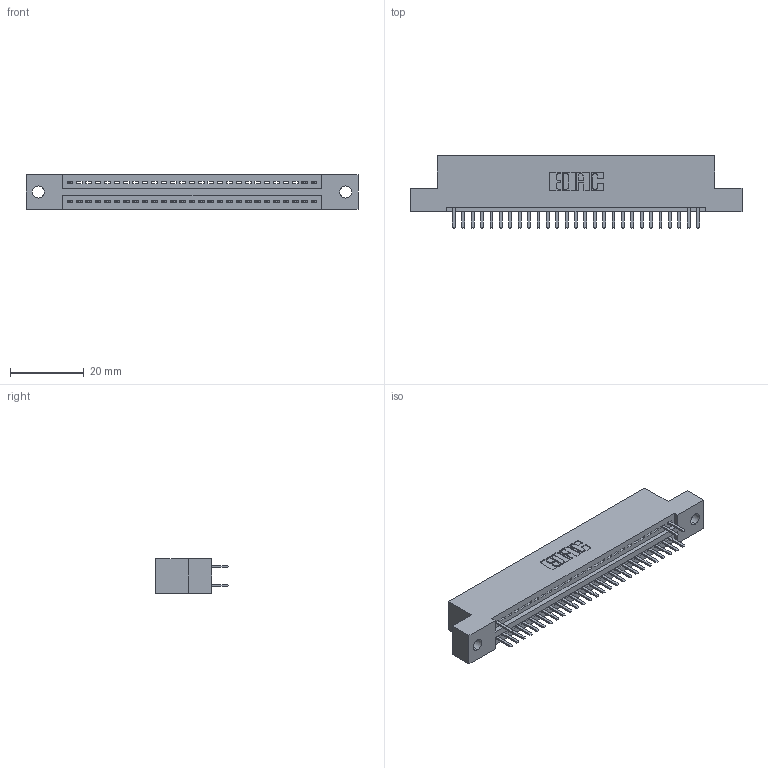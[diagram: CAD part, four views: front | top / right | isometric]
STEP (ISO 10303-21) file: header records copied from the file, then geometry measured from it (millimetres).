
FILE_DESCRIPTION (( 'STEP AP203' ), '1' );
FILE_NAME ('345-054-520-202.STEP', '2018-09-23T20:13:10', ( '' ), ( '' ), 'SwSTEP 2.0', 'SolidWorks 2016', '' );
FILE_SCHEMA (( 'CONFIG_CONTROL_DESIGN' ));
Length unit declared in the file: inch
Products named in the file (3): 345 Part_Flush Mounting Lugs - 0.128 Dia; 345-292-001_345-293-120; 345-054-520-202
Assembly tree (31 placements, depth 2):
  345-054-520-202
    345 Part_Flush Mounting Lugs - 0.128 Dia
    345-292-001_345-293-120  x30
Bounding box: 89.79 x 19.68 x 9.4 mm (x, y, z)
Volume: 8316.7 mm3; surface area: 10477 mm2
Topology: 31 solids, 31 shells, 1938 faces, 5699 edges, 3718 vertices
Faces by surface type: plane 1298, cylinder 640
Entity records: 22553 total; most frequent: CARTESIAN_POINT 3912, ORIENTED_EDGE 3858, DIRECTION 3429, EDGE_CURVE 1929, VECTOR 1685, LINE 1685, VERTEX_POINT 1282, AXIS2_PLACEMENT_3D 872
